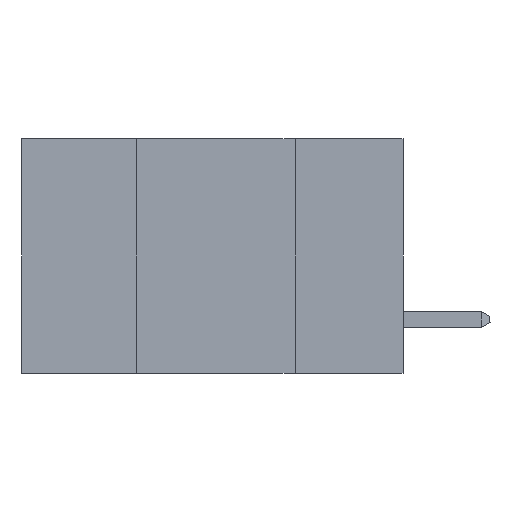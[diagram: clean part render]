
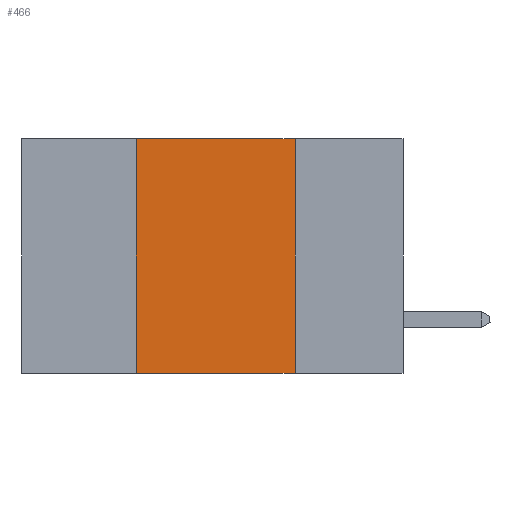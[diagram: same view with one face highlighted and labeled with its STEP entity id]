
A CAD part, left-side view. The second image highlights one B-rep face of the part: STEP entity #466.
In plain terms, the highlighted planar face has unit normal (-1, 0, 0).
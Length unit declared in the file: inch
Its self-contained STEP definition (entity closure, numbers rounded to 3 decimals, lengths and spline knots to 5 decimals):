
#466 = ADVANCED_FACE ( 'NONE', ( #5949 ), #5491, .F. ) ;
#636 = DIRECTION ( 'NONE',  ( 0., 0., -1. ) ) ;
#648 = VERTEX_POINT ( 'NONE', #2310 ) ;
#732 = EDGE_CURVE ( 'NONE', #6923, #13580, #2546, .T. ) ;
#1133 = CARTESIAN_POINT ( 'NONE',  ( 0., 0.17, 0. ) ) ;
#1363 = CARTESIAN_POINT ( 'NONE',  ( 0., 0.6, -0.37 ) ) ;
#1813 = CARTESIAN_POINT ( 'NONE',  ( 0., 0.6, 0. ) ) ;
#2265 = DIRECTION ( 'NONE',  ( 0., -1., 0. ) ) ;
#2278 = ORIENTED_EDGE ( 'NONE', *, *, #732, .F. ) ;
#2310 = CARTESIAN_POINT ( 'NONE',  ( 0., 0.42, -0.37 ) ) ;
#2521 = CARTESIAN_POINT ( 'NONE',  ( 0., 0.42, 0. ) ) ;
#2546 = LINE ( 'NONE', #15614, #10534 ) ;
#3007 = CARTESIAN_POINT ( 'NONE',  ( 0., 0.17, 0. ) ) ;
#3026 = VECTOR ( 'NONE', #12585, 39.37008 ) ;
#4064 = VECTOR ( 'NONE', #8597, 39.37008 ) ;
#4758 = DIRECTION ( 'NONE',  ( 0., -1., 0. ) ) ;
#5491 = PLANE ( 'NONE',  #13303 ) ;
#5949 = FACE_OUTER_BOUND ( 'NONE', #15217, .T. ) ;
#6923 = VERTEX_POINT ( 'NONE', #11147 ) ;
#7290 = LINE ( 'NONE', #2521, #4064 ) ;
#8569 = ORIENTED_EDGE ( 'NONE', *, *, #11033, .F. ) ;
#8597 = DIRECTION ( 'NONE',  ( 0., 0., 1. ) ) ;
#9730 = ORIENTED_EDGE ( 'NONE', *, *, #12829, .F. ) ;
#10291 = DIRECTION ( 'NONE',  ( 1., 0., 0. ) ) ;
#10396 = LINE ( 'NONE', #1363, #15303 ) ;
#10534 = VECTOR ( 'NONE', #2265, 39.37008 ) ;
#10590 = VERTEX_POINT ( 'NONE', #11646 ) ;
#11033 = EDGE_CURVE ( 'NONE', #13580, #10590, #11177, .T. ) ;
#11147 = CARTESIAN_POINT ( 'NONE',  ( 0., 0.42, 0. ) ) ;
#11177 = LINE ( 'NONE', #3007, #3026 ) ;
#11646 = CARTESIAN_POINT ( 'NONE',  ( 0., 0.17, -0.37 ) ) ;
#12585 = DIRECTION ( 'NONE',  ( 0., 0., -1. ) ) ;
#12829 = EDGE_CURVE ( 'NONE', #648, #6923, #7290, .T. ) ;
#13303 = AXIS2_PLACEMENT_3D ( 'NONE', #1813, #10291, #636 ) ;
#13373 = ORIENTED_EDGE ( 'NONE', *, *, #14632, .T. ) ;
#13580 = VERTEX_POINT ( 'NONE', #1133 ) ;
#14632 = EDGE_CURVE ( 'NONE', #648, #10590, #10396, .T. ) ;
#15217 = EDGE_LOOP ( 'NONE', ( #8569, #2278, #9730, #13373 ) ) ;
#15303 = VECTOR ( 'NONE', #4758, 39.37008 ) ;
#15614 = CARTESIAN_POINT ( 'NONE',  ( 0., 0.6, 0. ) ) ;
